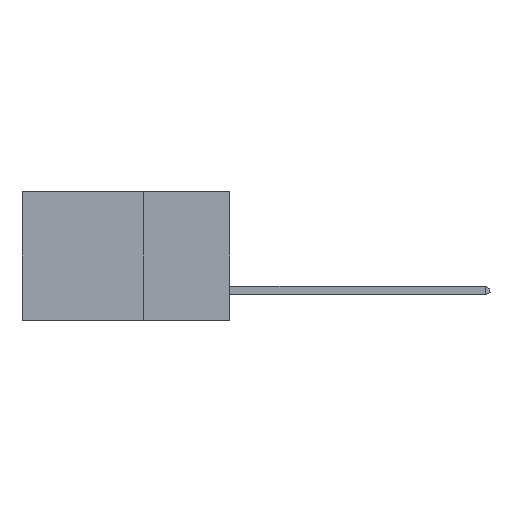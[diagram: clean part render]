
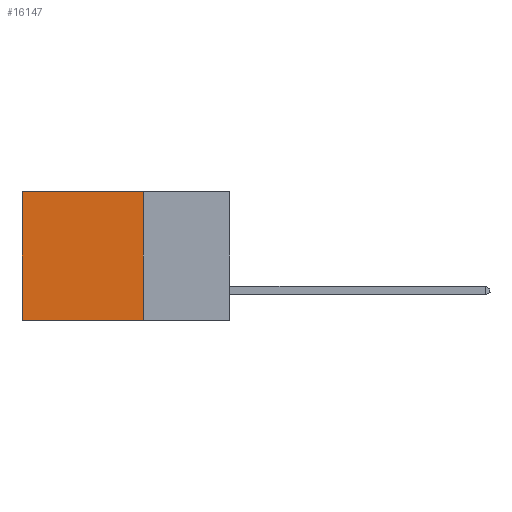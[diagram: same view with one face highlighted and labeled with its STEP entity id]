
A CAD part, left-side view. The second image highlights one B-rep face of the part: STEP entity #16147.
In plain terms, the highlighted planar face has unit normal (-1, 0, 0).
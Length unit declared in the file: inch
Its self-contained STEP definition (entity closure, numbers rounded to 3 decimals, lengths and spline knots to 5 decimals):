
#387 = ORIENTED_EDGE ( 'NONE', *, *, #8271, .T. ) ;
#941 = ORIENTED_EDGE ( 'NONE', *, *, #3593, .F. ) ;
#1236 = VERTEX_POINT ( 'NONE', #10252 ) ;
#1389 = AXIS2_PLACEMENT_3D ( 'NONE', #2911, #12031, #14541 ) ;
#1897 = CARTESIAN_POINT ( 'NONE',  ( 0.298, 0.25, 0. ) ) ;
#2530 = DIRECTION ( 'NONE',  ( 0., 0., -1. ) ) ;
#2838 = DIRECTION ( 'NONE',  ( 0., 0., -1. ) ) ;
#2911 = CARTESIAN_POINT ( 'NONE',  ( 0.298, 0.25, 0. ) ) ;
#2957 = FACE_OUTER_BOUND ( 'NONE', #5031, .T. ) ;
#3024 = EDGE_CURVE ( 'NONE', #12171, #10518, #3279, .T. ) ;
#3232 = ORIENTED_EDGE ( 'NONE', *, *, #15686, .T. ) ;
#3264 = LINE ( 'NONE', #7874, #13940 ) ;
#3279 = LINE ( 'NONE', #10388, #14558 ) ;
#3593 = EDGE_CURVE ( 'NONE', #10518, #4261, #3264, .T. ) ;
#3629 = ORIENTED_EDGE ( 'NONE', *, *, #3024, .F. ) ;
#4151 = DIRECTION ( 'NONE',  ( 0., 1., 0. ) ) ;
#4261 = VERTEX_POINT ( 'NONE', #8846 ) ;
#5031 = EDGE_LOOP ( 'NONE', ( #387, #941, #3629, #3232 ) ) ;
#5525 = CARTESIAN_POINT ( 'NONE',  ( 0.298, 0.6, 0. ) ) ;
#7794 = CARTESIAN_POINT ( 'NONE',  ( 0.298, 0.25, -0.37 ) ) ;
#7874 = CARTESIAN_POINT ( 'NONE',  ( 0.298, 0.25, -0.37 ) ) ;
#8271 = EDGE_CURVE ( 'NONE', #1236, #4261, #8394, .T. ) ;
#8394 = LINE ( 'NONE', #5525, #15573 ) ;
#8846 = CARTESIAN_POINT ( 'NONE',  ( 0.298, 0.6, -0.37 ) ) ;
#10252 = CARTESIAN_POINT ( 'NONE',  ( 0.298, 0.6, 0. ) ) ;
#10362 = LINE ( 'NONE', #1897, #14669 ) ;
#10388 = CARTESIAN_POINT ( 'NONE',  ( 0.298, 0.25, 0. ) ) ;
#10518 = VERTEX_POINT ( 'NONE', #7794 ) ;
#10824 = PLANE ( 'NONE',  #1389 ) ;
#12031 = DIRECTION ( 'NONE',  ( 1., 0., 0. ) ) ;
#12171 = VERTEX_POINT ( 'NONE', #14618 ) ;
#13756 = DIRECTION ( 'NONE',  ( 0., 1., 0. ) ) ;
#13940 = VECTOR ( 'NONE', #4151, 39.37008 ) ;
#14541 = DIRECTION ( 'NONE',  ( 0., 0., -1. ) ) ;
#14558 = VECTOR ( 'NONE', #2530, 39.37008 ) ;
#14618 = CARTESIAN_POINT ( 'NONE',  ( 0.298, 0.25, 0. ) ) ;
#14669 = VECTOR ( 'NONE', #13756, 39.37008 ) ;
#15573 = VECTOR ( 'NONE', #2838, 39.37008 ) ;
#15686 = EDGE_CURVE ( 'NONE', #12171, #1236, #10362, .T. ) ;
#16147 = ADVANCED_FACE ( 'NONE', ( #2957 ), #10824, .F. ) ;
